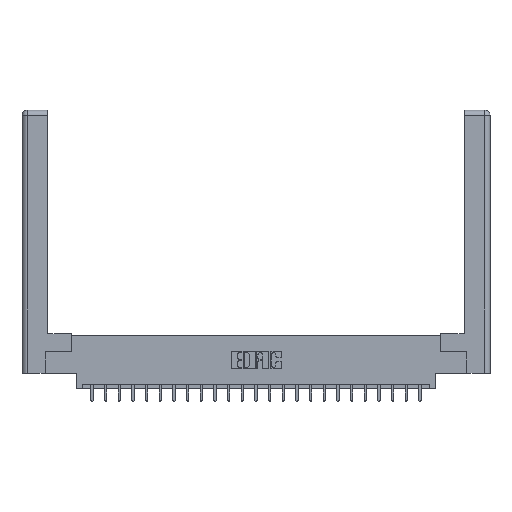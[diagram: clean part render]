
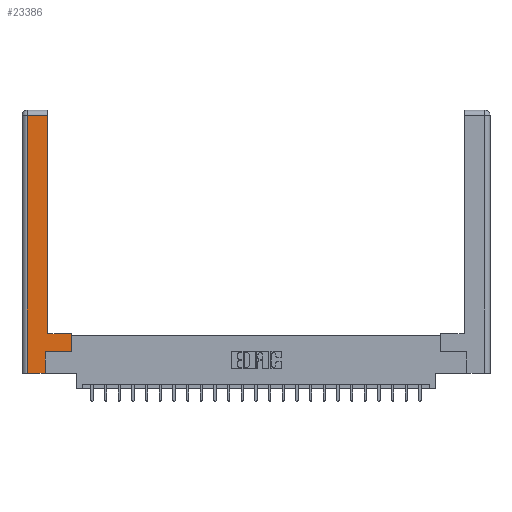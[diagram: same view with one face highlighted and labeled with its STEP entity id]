
A CAD part, top view. The second image highlights one B-rep face of the part: STEP entity #23386.
In plain terms, the highlighted planar face has unit normal (0, 0, 1).
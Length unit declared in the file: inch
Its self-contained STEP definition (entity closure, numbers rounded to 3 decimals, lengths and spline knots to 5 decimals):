
#313 = CARTESIAN_POINT ( 'NONE',  ( 0.295, 0.45, 0. ) ) ;
#394 = ORIENTED_EDGE ( 'NONE', *, *, #8003, .T. ) ;
#553 = EDGE_LOOP ( 'NONE', ( #13247, #20794, #4978, #9509, #22315, #4832, #10070, #394 ) ) ;
#1183 = LINE ( 'NONE', #1547, #2025 ) ;
#1494 = VERTEX_POINT ( 'NONE', #21619 ) ;
#1547 = CARTESIAN_POINT ( 'NONE',  ( 0.295, 0.45, 0. ) ) ;
#2025 = VECTOR ( 'NONE', #23854, 39.37008 ) ;
#2094 = EDGE_CURVE ( 'NONE', #5407, #10167, #12223, .T. ) ;
#2694 = CARTESIAN_POINT ( 'NONE',  ( 0.265, 0.245, 0. ) ) ;
#2884 = DIRECTION ( 'NONE',  ( 0., -1., 0. ) ) ;
#3095 = VECTOR ( 'NONE', #16924, 39.37008 ) ;
#3543 = VERTEX_POINT ( 'NONE', #20299 ) ;
#4586 = VECTOR ( 'NONE', #14618, 39.37008 ) ;
#4832 = ORIENTED_EDGE ( 'NONE', *, *, #12804, .T. ) ;
#4978 = ORIENTED_EDGE ( 'NONE', *, *, #2094, .T. ) ;
#5187 = LINE ( 'NONE', #7043, #15817 ) ;
#5393 = LINE ( 'NONE', #6281, #21883 ) ;
#5407 = VERTEX_POINT ( 'NONE', #10449 ) ;
#5820 = DIRECTION ( 'NONE',  ( 1., 0., 0. ) ) ;
#6203 = CARTESIAN_POINT ( 'NONE',  ( 0.0615, 0., 0. ) ) ;
#6281 = CARTESIAN_POINT ( 'NONE',  ( 0.0615, 2.94, 0. ) ) ;
#6430 = EDGE_CURVE ( 'NONE', #3543, #19136, #23023, .T. ) ;
#6913 = CARTESIAN_POINT ( 'NONE',  ( 0.0615, 0., 0. ) ) ;
#7043 = CARTESIAN_POINT ( 'NONE',  ( 0.265, 0.245, 0. ) ) ;
#7545 = VERTEX_POINT ( 'NONE', #10546 ) ;
#8003 = EDGE_CURVE ( 'NONE', #19136, #18387, #1183, .T. ) ;
#8200 = FACE_OUTER_BOUND ( 'NONE', #553, .T. ) ;
#9040 = VECTOR ( 'NONE', #5820, 39.37008 ) ;
#9351 = EDGE_CURVE ( 'NONE', #7545, #21941, #5187, .T. ) ;
#9411 = EDGE_CURVE ( 'NONE', #18387, #1494, #9653, .T. ) ;
#9509 = ORIENTED_EDGE ( 'NONE', *, *, #10378, .T. ) ;
#9572 = CARTESIAN_POINT ( 'NONE',  ( 0.565, 0.45, 0. ) ) ;
#9653 = LINE ( 'NONE', #11020, #4586 ) ;
#10070 = ORIENTED_EDGE ( 'NONE', *, *, #6430, .T. ) ;
#10083 = DIRECTION ( 'NONE',  ( -1., 0., 0. ) ) ;
#10167 = VERTEX_POINT ( 'NONE', #6913 ) ;
#10378 = EDGE_CURVE ( 'NONE', #10167, #7545, #14610, .T. ) ;
#10449 = CARTESIAN_POINT ( 'NONE',  ( 0.0615, 2.94, 0. ) ) ;
#10546 = CARTESIAN_POINT ( 'NONE',  ( 0.265, 0., 0. ) ) ;
#11020 = CARTESIAN_POINT ( 'NONE',  ( 0.295, 3., 0. ) ) ;
#11581 = EDGE_CURVE ( 'NONE', #1494, #5407, #5393, .T. ) ;
#11821 = VECTOR ( 'NONE', #18605, 39.37008 ) ;
#12223 = LINE ( 'NONE', #6203, #19248 ) ;
#12804 = EDGE_CURVE ( 'NONE', #21941, #3543, #17866, .T. ) ;
#13247 = ORIENTED_EDGE ( 'NONE', *, *, #9411, .T. ) ;
#14610 = LINE ( 'NONE', #17419, #9040 ) ;
#14618 = DIRECTION ( 'NONE',  ( 0., 1., 0. ) ) ;
#15817 = VECTOR ( 'NONE', #20428, 39.37008 ) ;
#16351 = CARTESIAN_POINT ( 'NONE',  ( 0., 0., 0. ) ) ;
#16924 = DIRECTION ( 'NONE',  ( 1., 0., 0. ) ) ;
#17419 = CARTESIAN_POINT ( 'NONE',  ( 0.265, 0., 0. ) ) ;
#17866 = LINE ( 'NONE', #24325, #3095 ) ;
#18387 = VERTEX_POINT ( 'NONE', #313 ) ;
#18605 = DIRECTION ( 'NONE',  ( 0., 1., 0. ) ) ;
#19033 = AXIS2_PLACEMENT_3D ( 'NONE', #16351, #19879, #23682 ) ;
#19136 = VERTEX_POINT ( 'NONE', #19195 ) ;
#19195 = CARTESIAN_POINT ( 'NONE',  ( 0.565, 0.45, 0. ) ) ;
#19248 = VECTOR ( 'NONE', #2884, 39.37008 ) ;
#19879 = DIRECTION ( 'NONE',  ( 0., 0., -1. ) ) ;
#20299 = CARTESIAN_POINT ( 'NONE',  ( 0.565, 0.245, 0. ) ) ;
#20428 = DIRECTION ( 'NONE',  ( 0., 1., 0. ) ) ;
#20794 = ORIENTED_EDGE ( 'NONE', *, *, #11581, .T. ) ;
#21619 = CARTESIAN_POINT ( 'NONE',  ( 0.295, 2.94, 0. ) ) ;
#21710 = PLANE ( 'NONE',  #19033 ) ;
#21883 = VECTOR ( 'NONE', #10083, 39.37008 ) ;
#21941 = VERTEX_POINT ( 'NONE', #2694 ) ;
#22315 = ORIENTED_EDGE ( 'NONE', *, *, #9351, .T. ) ;
#23023 = LINE ( 'NONE', #9572, #11821 ) ;
#23386 = ADVANCED_FACE ( 'NONE', ( #8200 ), #21710, .F. ) ;
#23682 = DIRECTION ( 'NONE',  ( -1., 0., 0. ) ) ;
#23854 = DIRECTION ( 'NONE',  ( -1., 0., 0. ) ) ;
#24325 = CARTESIAN_POINT ( 'NONE',  ( 0.565, 0.245, 0. ) ) ;
